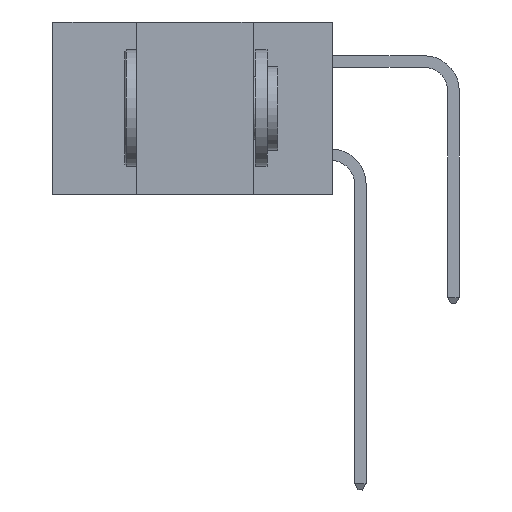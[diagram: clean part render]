
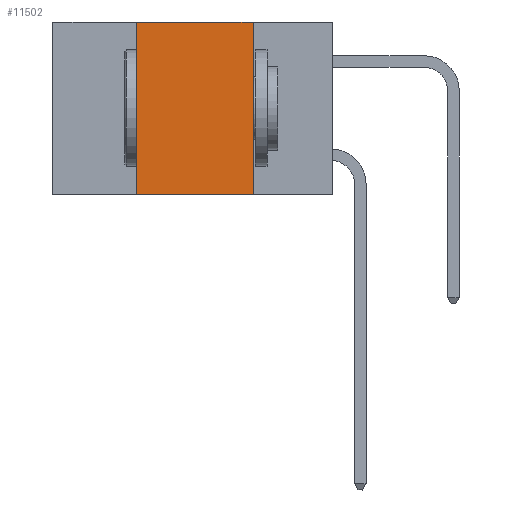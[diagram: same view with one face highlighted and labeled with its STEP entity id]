
A CAD part, left-side view. The second image highlights one B-rep face of the part: STEP entity #11502.
In plain terms, the highlighted planar face has unit normal (-1, 0, 0).
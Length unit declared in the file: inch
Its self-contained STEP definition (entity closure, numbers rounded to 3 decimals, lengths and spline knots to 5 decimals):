
#126 = CARTESIAN_POINT ( 'NONE',  ( 0., 0.17, -0.37 ) ) ;
#423 = CARTESIAN_POINT ( 'NONE',  ( 0., 0.6, -0.37 ) ) ;
#749 = CARTESIAN_POINT ( 'NONE',  ( 0., 0.6, 0. ) ) ;
#881 = DIRECTION ( 'NONE',  ( 1., 0., 0. ) ) ;
#1235 = CARTESIAN_POINT ( 'NONE',  ( 0., 0.6, 0. ) ) ;
#2364 = CARTESIAN_POINT ( 'NONE',  ( 0., 0.17, 0. ) ) ;
#2589 = CARTESIAN_POINT ( 'NONE',  ( 0., 0.17, -0.37 ) ) ;
#3509 = ORIENTED_EDGE ( 'NONE', *, *, #7455, .F. ) ;
#3705 = DIRECTION ( 'NONE',  ( 0., 0., -1. ) ) ;
#3749 = ORIENTED_EDGE ( 'NONE', *, *, #12142, .T. ) ;
#3981 = VERTEX_POINT ( 'NONE', #8046 ) ;
#4101 = EDGE_CURVE ( 'NONE', #8224, #5219, #11235, .T. ) ;
#4241 = DIRECTION ( 'NONE',  ( 0., -1., 0. ) ) ;
#4254 = LINE ( 'NONE', #423, #9902 ) ;
#4639 = DIRECTION ( 'NONE',  ( 0., 0., -1. ) ) ;
#5219 = VERTEX_POINT ( 'NONE', #126 ) ;
#5611 = DIRECTION ( 'NONE',  ( 0., 0., 1. ) ) ;
#6392 = DIRECTION ( 'NONE',  ( 0., -1., 0. ) ) ;
#6650 = CARTESIAN_POINT ( 'NONE',  ( 0., 0.42, -0.37 ) ) ;
#6709 = LINE ( 'NONE', #6650, #10451 ) ;
#7014 = VECTOR ( 'NONE', #4241, 39.37008 ) ;
#7356 = VECTOR ( 'NONE', #4639, 39.37008 ) ;
#7455 = EDGE_CURVE ( 'NONE', #9517, #3981, #6709, .T. ) ;
#8040 = LINE ( 'NONE', #1235, #7014 ) ;
#8046 = CARTESIAN_POINT ( 'NONE',  ( 0., 0.42, 0. ) ) ;
#8224 = VERTEX_POINT ( 'NONE', #2364 ) ;
#8339 = CARTESIAN_POINT ( 'NONE',  ( 0., 0.42, -0.37 ) ) ;
#8426 = ORIENTED_EDGE ( 'NONE', *, *, #4101, .F. ) ;
#9334 = ORIENTED_EDGE ( 'NONE', *, *, #10413, .F. ) ;
#9517 = VERTEX_POINT ( 'NONE', #8339 ) ;
#9555 = PLANE ( 'NONE',  #11696 ) ;
#9902 = VECTOR ( 'NONE', #6392, 39.37008 ) ;
#10413 = EDGE_CURVE ( 'NONE', #3981, #8224, #8040, .T. ) ;
#10451 = VECTOR ( 'NONE', #5611, 39.37008 ) ;
#11235 = LINE ( 'NONE', #2589, #7356 ) ;
#11371 = FACE_OUTER_BOUND ( 'NONE', #12135, .T. ) ;
#11502 = ADVANCED_FACE ( 'NONE', ( #11371 ), #9555, .F. ) ;
#11696 = AXIS2_PLACEMENT_3D ( 'NONE', #749, #881, #3705 ) ;
#12135 = EDGE_LOOP ( 'NONE', ( #8426, #9334, #3509, #3749 ) ) ;
#12142 = EDGE_CURVE ( 'NONE', #9517, #5219, #4254, .T. ) ;
